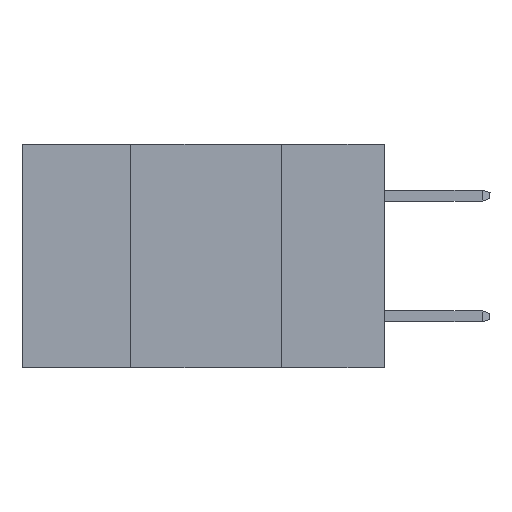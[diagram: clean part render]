
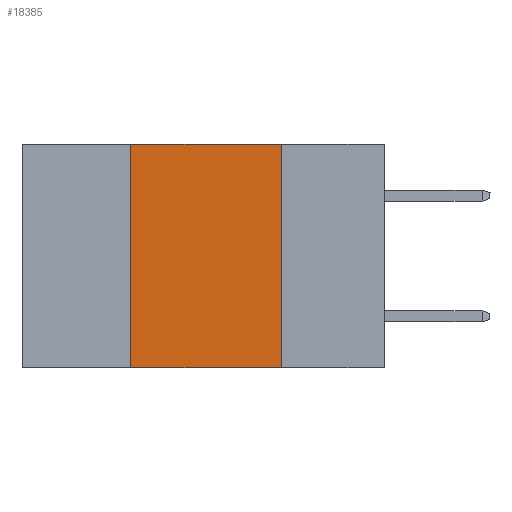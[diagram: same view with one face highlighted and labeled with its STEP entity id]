
A CAD part, left-side view. The second image highlights one B-rep face of the part: STEP entity #18385.
In plain terms, the highlighted planar face has unit normal (-1, 0, 0).
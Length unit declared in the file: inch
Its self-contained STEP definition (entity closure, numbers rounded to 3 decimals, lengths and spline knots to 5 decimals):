
#78 = ORIENTED_EDGE ( 'NONE', *, *, #7083, .F. ) ;
#909 = DIRECTION ( 'NONE',  ( 0., -1., 0. ) ) ;
#1209 = ORIENTED_EDGE ( 'NONE', *, *, #15790, .F. ) ;
#1769 = PLANE ( 'NONE',  #3159 ) ;
#1838 = LINE ( 'NONE', #15292, #14549 ) ;
#1861 = VECTOR ( 'NONE', #909, 39.37008 ) ;
#2491 = CARTESIAN_POINT ( 'NONE',  ( 0., 0.6, -0.37 ) ) ;
#2659 = EDGE_CURVE ( 'NONE', #6205, #18719, #19203, .T. ) ;
#2877 = CARTESIAN_POINT ( 'NONE',  ( 0., 0.17, 0. ) ) ;
#2951 = CARTESIAN_POINT ( 'NONE',  ( 0., 0.42, -0.37 ) ) ;
#3159 = AXIS2_PLACEMENT_3D ( 'NONE', #13133, #9879, #9815 ) ;
#3937 = ORIENTED_EDGE ( 'NONE', *, *, #17431, .F. ) ;
#4393 = DIRECTION ( 'NONE',  ( 0., -1., 0. ) ) ;
#4528 = DIRECTION ( 'NONE',  ( 0., 0., -1. ) ) ;
#4981 = EDGE_LOOP ( 'NONE', ( #1209, #3937, #78, #19008 ) ) ;
#6018 = CARTESIAN_POINT ( 'NONE',  ( 0., 0.17, 0. ) ) ;
#6205 = VERTEX_POINT ( 'NONE', #2951 ) ;
#7083 = EDGE_CURVE ( 'NONE', #6205, #10286, #1838, .T. ) ;
#7526 = CARTESIAN_POINT ( 'NONE',  ( 0., 0.42, 0. ) ) ;
#9273 = CARTESIAN_POINT ( 'NONE',  ( 0., 0.6, 0. ) ) ;
#9815 = DIRECTION ( 'NONE',  ( 0., 0., -1. ) ) ;
#9879 = DIRECTION ( 'NONE',  ( 1., 0., 0. ) ) ;
#10260 = LINE ( 'NONE', #9273, #18998 ) ;
#10286 = VERTEX_POINT ( 'NONE', #7526 ) ;
#13133 = CARTESIAN_POINT ( 'NONE',  ( 0., 0.6, 0. ) ) ;
#13888 = VECTOR ( 'NONE', #4528, 39.37008 ) ;
#14549 = VECTOR ( 'NONE', #15650, 39.37008 ) ;
#14704 = FACE_OUTER_BOUND ( 'NONE', #4981, .T. ) ;
#15292 = CARTESIAN_POINT ( 'NONE',  ( 0., 0.42, 0. ) ) ;
#15650 = DIRECTION ( 'NONE',  ( 0., 0., 1. ) ) ;
#15790 = EDGE_CURVE ( 'NONE', #16564, #18719, #17792, .T. ) ;
#16564 = VERTEX_POINT ( 'NONE', #6018 ) ;
#17431 = EDGE_CURVE ( 'NONE', #10286, #16564, #10260, .T. ) ;
#17792 = LINE ( 'NONE', #2877, #13888 ) ;
#18385 = ADVANCED_FACE ( 'NONE', ( #14704 ), #1769, .F. ) ;
#18719 = VERTEX_POINT ( 'NONE', #18891 ) ;
#18891 = CARTESIAN_POINT ( 'NONE',  ( 0., 0.17, -0.37 ) ) ;
#18998 = VECTOR ( 'NONE', #4393, 39.37008 ) ;
#19008 = ORIENTED_EDGE ( 'NONE', *, *, #2659, .T. ) ;
#19203 = LINE ( 'NONE', #2491, #1861 ) ;
